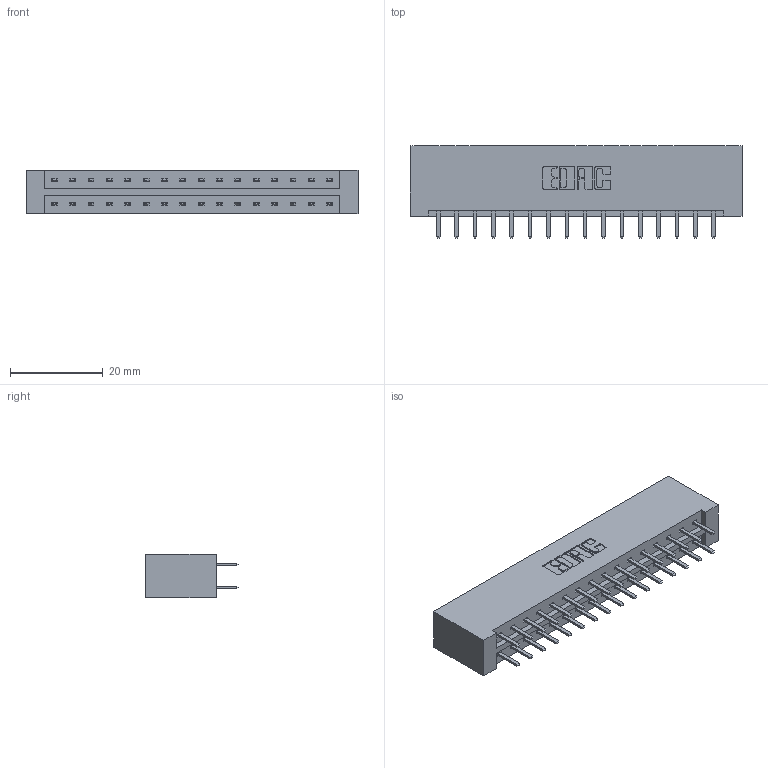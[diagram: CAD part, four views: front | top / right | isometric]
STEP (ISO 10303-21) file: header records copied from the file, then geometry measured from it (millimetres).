
FILE_DESCRIPTION (( 'STEP AP203' ), '1' );
FILE_NAME ('333-032-520-201.STEP', '2018-08-02T19:42:34', ( '' ), ( '' ), 'SwSTEP 2.0', 'SolidWorks 2016', '' );
FILE_SCHEMA (( 'CONFIG_CONTROL_DESIGN' ));
Length unit declared in the file: inch
Products named in the file (3): 333 Part_Lugless; 333-032-520-201; 345-292-001_345-293-120
Assembly tree (33 placements, depth 2):
  333-032-520-201
    333 Part_Lugless
    345-292-001_345-293-120  x32
Bounding box: 71.65 x 20.02 x 9.4 mm (x, y, z)
Volume: 7690.4 mm3; surface area: 8799.7 mm2
Topology: 33 solids, 33 shells, 1898 faces, 5503 edges, 3582 vertices
Faces by surface type: plane 1282, cylinder 616
Entity records: 13493 total; most frequent: CARTESIAN_POINT 2278, ORIENTED_EDGE 2202, DIRECTION 1973, EDGE_CURVE 1101, VECTOR 977, LINE 977, VERTEX_POINT 730, AXIS2_PLACEMENT_3D 498
